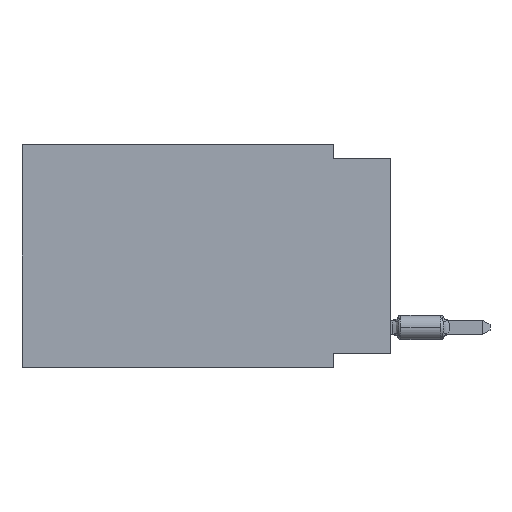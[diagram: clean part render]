
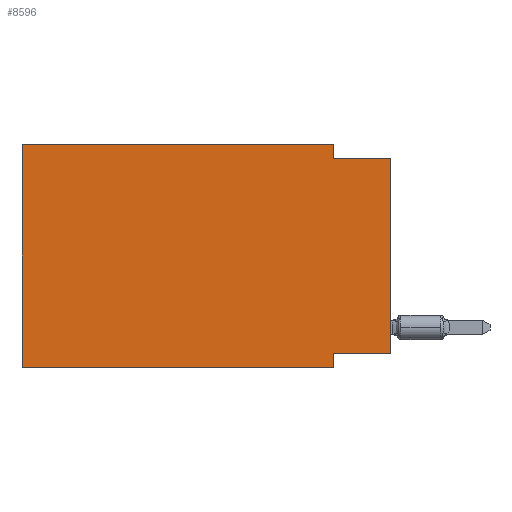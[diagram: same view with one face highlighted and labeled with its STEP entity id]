
A CAD part, left-side view. The second image highlights one B-rep face of the part: STEP entity #8596.
In plain terms, the highlighted planar face has unit normal (-1, 0, 0).
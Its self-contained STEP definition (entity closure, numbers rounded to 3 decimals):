
#284 = VERTEX_POINT ( 'NONE', #7576 ) ;
#696 = ORIENTED_EDGE ( 'NONE', *, *, #1679, .F. ) ;
#1274 = LINE ( 'NONE', #8667, #12479 ) ;
#1679 = EDGE_CURVE ( 'NONE', #4908, #14434, #1274, .T. ) ;
#2171 = ORIENTED_EDGE ( 'NONE', *, *, #15903, .F. ) ;
#2251 = EDGE_CURVE ( 'NONE', #9916, #14434, #15653, .T. ) ;
#2738 = EDGE_CURVE ( 'NONE', #17154, #10006, #5894, .T. ) ;
#2816 = ORIENTED_EDGE ( 'NONE', *, *, #2251, .T. ) ;
#3879 = VERTEX_POINT ( 'NONE', #9887 ) ;
#3896 = AXIS2_PLACEMENT_3D ( 'NONE', #10655, #7709, #16466 ) ;
#3949 = VERTEX_POINT ( 'NONE', #18023 ) ;
#4438 = LINE ( 'NONE', #4546, #6813 ) ;
#4546 = CARTESIAN_POINT ( 'NONE',  ( 0., 0., -0.635 ) ) ;
#4908 = VERTEX_POINT ( 'NONE', #7599 ) ;
#5378 = VECTOR ( 'NONE', #16868, 1000. ) ;
#5432 = VECTOR ( 'NONE', #15764, 1000. ) ;
#5816 = LINE ( 'NONE', #7201, #15661 ) ;
#5846 = ORIENTED_EDGE ( 'NONE', *, *, #10518, .F. ) ;
#5852 = CARTESIAN_POINT ( 'NONE',  ( 0., 2.54, 0. ) ) ;
#5894 = LINE ( 'NONE', #8390, #9757 ) ;
#6116 = EDGE_LOOP ( 'NONE', ( #12506, #5846, #15171, #6950, #11146, #2816, #696, #2171 ) ) ;
#6418 = CARTESIAN_POINT ( 'NONE',  ( 0., 0., -9.271 ) ) ;
#6813 = VECTOR ( 'NONE', #11369, 1000. ) ;
#6950 = ORIENTED_EDGE ( 'NONE', *, *, #10945, .F. ) ;
#7201 = CARTESIAN_POINT ( 'NONE',  ( 0., 16.383, 0. ) ) ;
#7576 = CARTESIAN_POINT ( 'NONE',  ( 0., 2.54, -0.635 ) ) ;
#7599 = CARTESIAN_POINT ( 'NONE',  ( 0., 2.54, -9.271 ) ) ;
#7632 = EDGE_CURVE ( 'NONE', #3949, #284, #17092, .T. ) ;
#7709 = DIRECTION ( 'NONE',  ( 1., 0., 0. ) ) ;
#7805 = CARTESIAN_POINT ( 'NONE',  ( 0., 0., -9.271 ) ) ;
#8390 = CARTESIAN_POINT ( 'NONE',  ( 0., 0., 0. ) ) ;
#8596 = ADVANCED_FACE ( 'NONE', ( #10830 ), #10575, .F. ) ;
#8667 = CARTESIAN_POINT ( 'NONE',  ( 0., 2.54, -9.906 ) ) ;
#9434 = LINE ( 'NONE', #6418, #11844 ) ;
#9757 = VECTOR ( 'NONE', #15774, 1000. ) ;
#9887 = CARTESIAN_POINT ( 'NONE',  ( 0., 16.383, 0. ) ) ;
#9916 = VERTEX_POINT ( 'NONE', #10202 ) ;
#10006 = VERTEX_POINT ( 'NONE', #14910 ) ;
#10084 = DIRECTION ( 'NONE',  ( 0., 0., -1. ) ) ;
#10124 = CARTESIAN_POINT ( 'NONE',  ( 0., 16.383, -9.906 ) ) ;
#10202 = CARTESIAN_POINT ( 'NONE',  ( 0., 16.383, -9.906 ) ) ;
#10491 = CARTESIAN_POINT ( 'NONE',  ( 0., 2.54, -9.906 ) ) ;
#10518 = EDGE_CURVE ( 'NONE', #284, #10006, #4438, .T. ) ;
#10575 = PLANE ( 'NONE',  #3896 ) ;
#10655 = CARTESIAN_POINT ( 'NONE',  ( 0., 16.383, 0. ) ) ;
#10830 = FACE_OUTER_BOUND ( 'NONE', #6116, .T. ) ;
#10945 = EDGE_CURVE ( 'NONE', #3879, #3949, #5816, .T. ) ;
#11146 = ORIENTED_EDGE ( 'NONE', *, *, #16464, .F. ) ;
#11369 = DIRECTION ( 'NONE',  ( 0., -1., 0. ) ) ;
#11844 = VECTOR ( 'NONE', #16285, 1000. ) ;
#12479 = VECTOR ( 'NONE', #14196, 1000. ) ;
#12506 = ORIENTED_EDGE ( 'NONE', *, *, #2738, .T. ) ;
#14196 = DIRECTION ( 'NONE',  ( 0., 0., -1. ) ) ;
#14294 = DIRECTION ( 'NONE',  ( 0., -1., 0. ) ) ;
#14434 = VERTEX_POINT ( 'NONE', #10491 ) ;
#14910 = CARTESIAN_POINT ( 'NONE',  ( 0., 0., -0.635 ) ) ;
#14965 = VECTOR ( 'NONE', #10084, 1000. ) ;
#15171 = ORIENTED_EDGE ( 'NONE', *, *, #7632, .F. ) ;
#15653 = LINE ( 'NONE', #10124, #5432 ) ;
#15660 = CARTESIAN_POINT ( 'NONE',  ( 0., 16.383, 0. ) ) ;
#15661 = VECTOR ( 'NONE', #14294, 1000. ) ;
#15764 = DIRECTION ( 'NONE',  ( 0., -1., 0. ) ) ;
#15774 = DIRECTION ( 'NONE',  ( 0., 0., 1. ) ) ;
#15903 = EDGE_CURVE ( 'NONE', #17154, #4908, #9434, .T. ) ;
#16285 = DIRECTION ( 'NONE',  ( 0., 1., 0. ) ) ;
#16464 = EDGE_CURVE ( 'NONE', #9916, #3879, #17130, .T. ) ;
#16466 = DIRECTION ( 'NONE',  ( 0., 0., -1. ) ) ;
#16868 = DIRECTION ( 'NONE',  ( 0., 0., 1. ) ) ;
#17092 = LINE ( 'NONE', #5852, #14965 ) ;
#17130 = LINE ( 'NONE', #15660, #5378 ) ;
#17154 = VERTEX_POINT ( 'NONE', #7805 ) ;
#18023 = CARTESIAN_POINT ( 'NONE',  ( 0., 2.54, 0. ) ) ;
